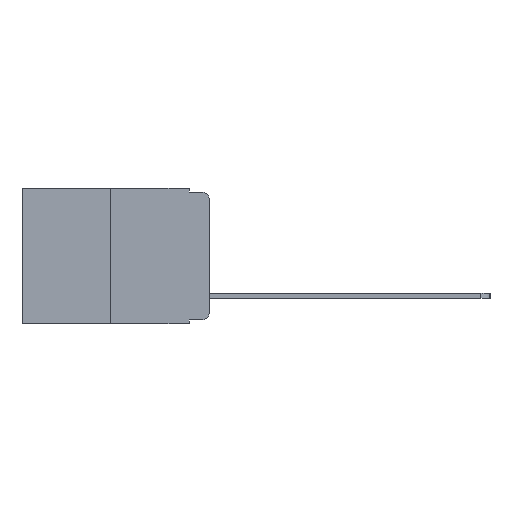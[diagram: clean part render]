
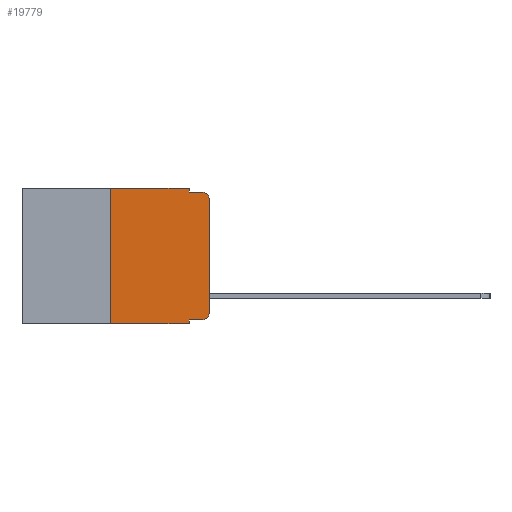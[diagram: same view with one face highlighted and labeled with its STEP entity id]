
A CAD part, left-side view. The second image highlights one B-rep face of the part: STEP entity #19779.
In plain terms, the highlighted planar face has unit normal (-1, 0, 0).
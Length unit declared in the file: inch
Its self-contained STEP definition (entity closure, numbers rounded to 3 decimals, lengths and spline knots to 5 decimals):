
#613 = CARTESIAN_POINT ( 'NONE',  ( 0., 0.051, -0.333 ) ) ;
#738 = VECTOR ( 'NONE', #22984, 39.37008 ) ;
#804 = DIRECTION ( 'NONE',  ( 0., 0., -1. ) ) ;
#840 = PLANE ( 'NONE',  #15513 ) ;
#858 = ORIENTED_EDGE ( 'NONE', *, *, #3882, .T. ) ;
#1160 = DIRECTION ( 'NONE',  ( 0., -1., 0. ) ) ;
#1162 = EDGE_CURVE ( 'NONE', #12418, #13614, #3973, .T. ) ;
#2743 = DIRECTION ( 'NONE',  ( 0., 0., -1. ) ) ;
#3209 = DIRECTION ( 'NONE',  ( -1., 0., 0. ) ) ;
#3443 = FACE_OUTER_BOUND ( 'NONE', #7942, .T. ) ;
#3882 = EDGE_CURVE ( 'NONE', #13614, #15654, #6537, .T. ) ;
#3973 = LINE ( 'NONE', #10542, #18665 ) ;
#4154 = ORIENTED_EDGE ( 'NONE', *, *, #16908, .F. ) ;
#4288 = VERTEX_POINT ( 'NONE', #23090 ) ;
#4358 = DIRECTION ( 'NONE',  ( 0., 0., 1. ) ) ;
#4537 = DIRECTION ( 'NONE',  ( 0., 0., 1. ) ) ;
#4676 = CARTESIAN_POINT ( 'NONE',  ( 0., 0.051, -0.01 ) ) ;
#5496 = ORIENTED_EDGE ( 'NONE', *, *, #18085, .F. ) ;
#5755 = ORIENTED_EDGE ( 'NONE', *, *, #10489, .T. ) ;
#6011 = CARTESIAN_POINT ( 'NONE',  ( 0., 0.051, 0. ) ) ;
#6103 = CARTESIAN_POINT ( 'NONE',  ( 0., 0.051, -0.01 ) ) ;
#6220 = CARTESIAN_POINT ( 'NONE',  ( 0., 0.25, -0.343 ) ) ;
#6537 = CIRCLE ( 'NONE', #6878, 0.02 ) ;
#6591 = CARTESIAN_POINT ( 'NONE',  ( 0., 0.473, 0. ) ) ;
#6878 = AXIS2_PLACEMENT_3D ( 'NONE', #24029, #12915, #22058 ) ;
#7062 = EDGE_CURVE ( 'NONE', #17415, #10009, #15912, .T. ) ;
#7338 = CARTESIAN_POINT ( 'NONE',  ( 0., 0., -0.313 ) ) ;
#7634 = LINE ( 'NONE', #6011, #738 ) ;
#7942 = EDGE_LOOP ( 'NONE', ( #5755, #19516, #5496, #20475, #18760, #15554, #13068, #4154, #20425, #858 ) ) ;
#8179 = VERTEX_POINT ( 'NONE', #13250 ) ;
#8311 = VECTOR ( 'NONE', #19927, 39.37008 ) ;
#8433 = DIRECTION ( 'NONE',  ( 0., -1., 0. ) ) ;
#8482 = LINE ( 'NONE', #23424, #23469 ) ;
#8483 = EDGE_CURVE ( 'NONE', #4288, #8179, #24424, .T. ) ;
#8944 = VERTEX_POINT ( 'NONE', #19249 ) ;
#9940 = VECTOR ( 'NONE', #804, 39.37008 ) ;
#10009 = VERTEX_POINT ( 'NONE', #19204 ) ;
#10489 = EDGE_CURVE ( 'NONE', #15654, #8944, #8482, .T. ) ;
#10542 = CARTESIAN_POINT ( 'NONE',  ( 0., 0.051, -0.333 ) ) ;
#12418 = VERTEX_POINT ( 'NONE', #613 ) ;
#12463 = DIRECTION ( 'NONE',  ( 0., -1., 0. ) ) ;
#12915 = DIRECTION ( 'NONE',  ( -1., 0., 0. ) ) ;
#13068 = ORIENTED_EDGE ( 'NONE', *, *, #7062, .T. ) ;
#13250 = CARTESIAN_POINT ( 'NONE',  ( 0., 0.051, 0. ) ) ;
#13614 = VERTEX_POINT ( 'NONE', #15709 ) ;
#14267 = DIRECTION ( 'NONE',  ( 1., 0., 0. ) ) ;
#14481 = CARTESIAN_POINT ( 'NONE',  ( 0., 0.02, -0.01 ) ) ;
#14538 = EDGE_CURVE ( 'NONE', #8944, #20608, #20189, .T. ) ;
#14577 = CARTESIAN_POINT ( 'NONE',  ( 0., 0.473, -0.343 ) ) ;
#14735 = CARTESIAN_POINT ( 'NONE',  ( 0., 0.02, -0.03 ) ) ;
#15063 = LINE ( 'NONE', #23444, #9940 ) ;
#15234 = EDGE_CURVE ( 'NONE', #8179, #21577, #7634, .T. ) ;
#15513 = AXIS2_PLACEMENT_3D ( 'NONE', #21584, #14267, #2743 ) ;
#15554 = ORIENTED_EDGE ( 'NONE', *, *, #19191, .F. ) ;
#15654 = VERTEX_POINT ( 'NONE', #7338 ) ;
#15709 = CARTESIAN_POINT ( 'NONE',  ( 0., 0.02, -0.333 ) ) ;
#15893 = CARTESIAN_POINT ( 'NONE',  ( 0., 0.25, 0. ) ) ;
#15912 = LINE ( 'NONE', #14577, #21385 ) ;
#16683 = DIRECTION ( 'NONE',  ( 0., 0., -1. ) ) ;
#16908 = EDGE_CURVE ( 'NONE', #12418, #10009, #15063, .T. ) ;
#17415 = VERTEX_POINT ( 'NONE', #6220 ) ;
#17576 = VECTOR ( 'NONE', #4358, 39.37008 ) ;
#18085 = EDGE_CURVE ( 'NONE', #21577, #20608, #22735, .T. ) ;
#18665 = VECTOR ( 'NONE', #12463, 39.37008 ) ;
#18760 = ORIENTED_EDGE ( 'NONE', *, *, #8483, .F. ) ;
#19191 = EDGE_CURVE ( 'NONE', #17415, #4288, #22390, .T. ) ;
#19204 = CARTESIAN_POINT ( 'NONE',  ( 0., 0.051, -0.343 ) ) ;
#19249 = CARTESIAN_POINT ( 'NONE',  ( 0., 0., -0.03 ) ) ;
#19516 = ORIENTED_EDGE ( 'NONE', *, *, #14538, .T. ) ;
#19779 = ADVANCED_FACE ( 'NONE', ( #3443 ), #840, .F. ) ;
#19927 = DIRECTION ( 'NONE',  ( 0., -1., 0. ) ) ;
#20189 = CIRCLE ( 'NONE', #22976, 0.02 ) ;
#20425 = ORIENTED_EDGE ( 'NONE', *, *, #1162, .T. ) ;
#20475 = ORIENTED_EDGE ( 'NONE', *, *, #15234, .F. ) ;
#20608 = VERTEX_POINT ( 'NONE', #14481 ) ;
#21385 = VECTOR ( 'NONE', #1160, 39.37008 ) ;
#21577 = VERTEX_POINT ( 'NONE', #6103 ) ;
#21584 = CARTESIAN_POINT ( 'NONE',  ( 0., 0.473, 0. ) ) ;
#22058 = DIRECTION ( 'NONE',  ( 0., 0., -1. ) ) ;
#22390 = LINE ( 'NONE', #15893, #17576 ) ;
#22735 = LINE ( 'NONE', #4676, #8311 ) ;
#22976 = AXIS2_PLACEMENT_3D ( 'NONE', #14735, #3209, #16683 ) ;
#22984 = DIRECTION ( 'NONE',  ( 0., 0., -1. ) ) ;
#23090 = CARTESIAN_POINT ( 'NONE',  ( 0., 0.25, 0. ) ) ;
#23424 = CARTESIAN_POINT ( 'NONE',  ( 0., 0., 0. ) ) ;
#23444 = CARTESIAN_POINT ( 'NONE',  ( 0., 0.051, 0. ) ) ;
#23469 = VECTOR ( 'NONE', #4537, 39.37008 ) ;
#23866 = VECTOR ( 'NONE', #8433, 39.37008 ) ;
#24029 = CARTESIAN_POINT ( 'NONE',  ( 0., 0.02, -0.313 ) ) ;
#24424 = LINE ( 'NONE', #6591, #23866 ) ;
